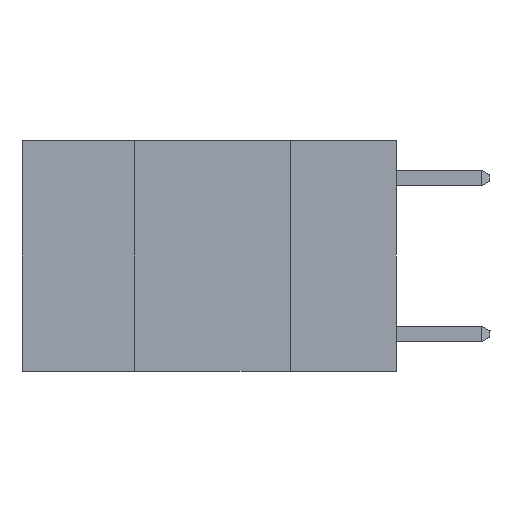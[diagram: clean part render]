
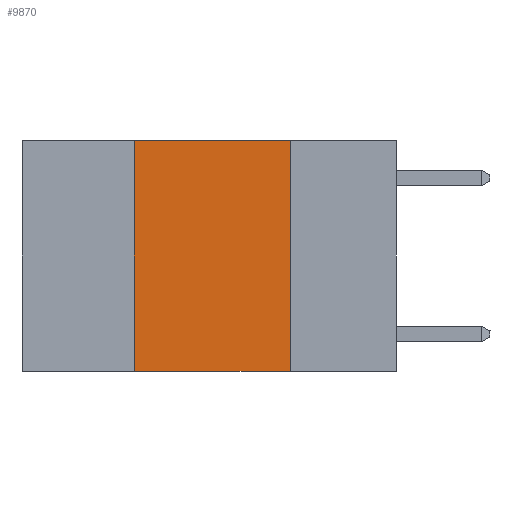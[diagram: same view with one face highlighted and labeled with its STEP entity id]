
A CAD part, left-side view. The second image highlights one B-rep face of the part: STEP entity #9870.
In plain terms, the highlighted planar face has unit normal (-1, 0, 0).
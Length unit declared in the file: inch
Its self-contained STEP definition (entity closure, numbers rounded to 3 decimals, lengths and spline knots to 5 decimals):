
#380 = VERTEX_POINT ( 'NONE', #6669 ) ;
#502 = DIRECTION ( 'NONE',  ( 1., 0., 0. ) ) ;
#538 = VERTEX_POINT ( 'NONE', #2977 ) ;
#539 = VERTEX_POINT ( 'NONE', #9273 ) ;
#951 = VECTOR ( 'NONE', #14682, 39.37008 ) ;
#1828 = ORIENTED_EDGE ( 'NONE', *, *, #11698, .F. ) ;
#2052 = LINE ( 'NONE', #6819, #951 ) ;
#2194 = VECTOR ( 'NONE', #14687, 39.37008 ) ;
#2493 = CARTESIAN_POINT ( 'NONE',  ( 0., 0.42, 0. ) ) ;
#2569 = LINE ( 'NONE', #7967, #2194 ) ;
#2977 = CARTESIAN_POINT ( 'NONE',  ( 0., 0.17, 0. ) ) ;
#3120 = AXIS2_PLACEMENT_3D ( 'NONE', #5118, #502, #8573 ) ;
#4704 = CARTESIAN_POINT ( 'NONE',  ( 0., 0.17, 0. ) ) ;
#5118 = CARTESIAN_POINT ( 'NONE',  ( 0., 0.6, 0. ) ) ;
#5705 = ORIENTED_EDGE ( 'NONE', *, *, #5711, .F. ) ;
#5711 = EDGE_CURVE ( 'NONE', #380, #538, #2052, .T. ) ;
#5860 = DIRECTION ( 'NONE',  ( 0., 0., -1. ) ) ;
#6190 = LINE ( 'NONE', #2493, #14487 ) ;
#6669 = CARTESIAN_POINT ( 'NONE',  ( 0., 0.42, 0. ) ) ;
#6780 = ORIENTED_EDGE ( 'NONE', *, *, #9627, .F. ) ;
#6819 = CARTESIAN_POINT ( 'NONE',  ( 0., 0.6, 0. ) ) ;
#6943 = ORIENTED_EDGE ( 'NONE', *, *, #12877, .T. ) ;
#7403 = PLANE ( 'NONE',  #3120 ) ;
#7967 = CARTESIAN_POINT ( 'NONE',  ( 0., 0.6, -0.37 ) ) ;
#8573 = DIRECTION ( 'NONE',  ( 0., 0., -1. ) ) ;
#8575 = VECTOR ( 'NONE', #5860, 39.37008 ) ;
#8925 = LINE ( 'NONE', #4704, #8575 ) ;
#9273 = CARTESIAN_POINT ( 'NONE',  ( 0., 0.17, -0.37 ) ) ;
#9627 = EDGE_CURVE ( 'NONE', #538, #539, #8925, .T. ) ;
#9870 = ADVANCED_FACE ( 'NONE', ( #14345 ), #7403, .F. ) ;
#10139 = CARTESIAN_POINT ( 'NONE',  ( 0., 0.42, -0.37 ) ) ;
#10275 = VERTEX_POINT ( 'NONE', #10139 ) ;
#11032 = EDGE_LOOP ( 'NONE', ( #6780, #5705, #1828, #6943 ) ) ;
#11698 = EDGE_CURVE ( 'NONE', #10275, #380, #6190, .T. ) ;
#12689 = DIRECTION ( 'NONE',  ( 0., 0., 1. ) ) ;
#12877 = EDGE_CURVE ( 'NONE', #10275, #539, #2569, .T. ) ;
#14345 = FACE_OUTER_BOUND ( 'NONE', #11032, .T. ) ;
#14487 = VECTOR ( 'NONE', #12689, 39.37008 ) ;
#14682 = DIRECTION ( 'NONE',  ( 0., -1., 0. ) ) ;
#14687 = DIRECTION ( 'NONE',  ( 0., -1., 0. ) ) ;
